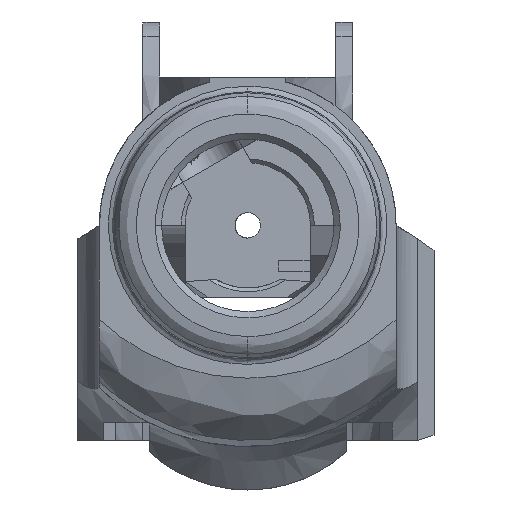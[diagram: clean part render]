
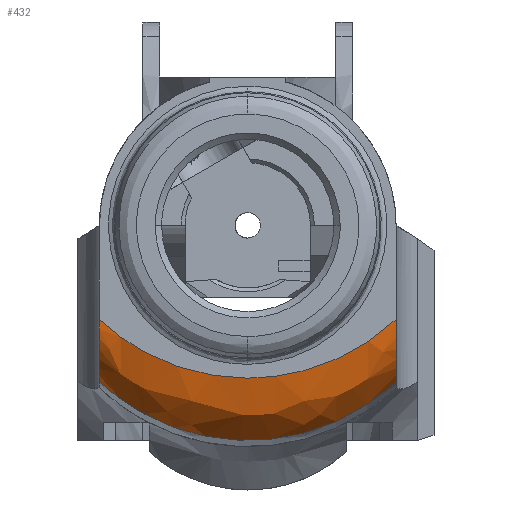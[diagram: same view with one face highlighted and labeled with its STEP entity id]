
A CAD part, left-side view. The second image highlights one B-rep face of the part: STEP entity #432.
In plain terms, the highlighted free-form (B-spline) face has degree [3, 3] with [4, 10] control points.
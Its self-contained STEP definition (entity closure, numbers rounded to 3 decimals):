
#432=ADVANCED_FACE('',(#892),#7309,.T.);
#892=FACE_OUTER_BOUND('',#1352,.T.);
#1352=EDGE_LOOP('',(#3797,#3798,#3799,#3800,#3801,#3802));
#3797=ORIENTED_EDGE('',*,*,#4130,.T.);
#3798=ORIENTED_EDGE('',*,*,#3877,.T.);
#3799=ORIENTED_EDGE('',*,*,#3878,.T.);
#3800=ORIENTED_EDGE('',*,*,#3879,.T.);
#3801=ORIENTED_EDGE('',*,*,#4136,.F.);
#3802=ORIENTED_EDGE('',*,*,#4133,.F.);
#3877=EDGE_CURVE('',#6382,#6383,#6224,.T.);
#3878=EDGE_CURVE('',#6383,#6384,#5129,.T.);
#3879=EDGE_CURVE('',#6384,#6385,#6225,.T.);
#4130=EDGE_CURVE('',#6630,#6382,#5347,.T.);
#4133=EDGE_CURVE('',#6630,#6631,#6259,.T.);
#4136=EDGE_CURVE('',#6631,#6385,#5352,.T.);
#5129=B_SPLINE_CURVE_WITH_KNOTS('',3,(#11458,#11459,#11460,#11461,#11462),
 .UNSPECIFIED.,.F.,.F.,(4,1,4),(0.,0.015,0.029),
 .UNSPECIFIED.);
#5347=B_SPLINE_CURVE_WITH_KNOTS('',3,(#12147,#12148,#12149,#12150,#12151,
#12152,#12153,#12154,#12155,#12156,#12157),.UNSPECIFIED.,.F.,.F.,(4,1,1,
1,1,1,1,1,4),(0.,0.77,1.54,2.311,3.081,
3.851,4.621,5.392,6.162),
 .UNSPECIFIED.);
#5352=B_SPLINE_CURVE_WITH_KNOTS('',3,(#12169,#12170,#12171,#12172,#12173,
#12174,#12175,#12176,#12177,#12178,#12179),.UNSPECIFIED.,.F.,.F.,(4,1,1,
1,1,1,1,1,4),(-6.162,-5.392,-4.621,-3.851,
-3.081,-2.311,-1.54,-0.77,
0.),.UNSPECIFIED.);
#6224=(
BOUNDED_CURVE()
B_SPLINE_CURVE(2,(#11455,#11456,#11457),.UNSPECIFIED.,.F.,.F.)
B_SPLINE_CURVE_WITH_KNOTS((3,3),(0.,12.819),.UNSPECIFIED.)
CURVE()
GEOMETRIC_REPRESENTATION_ITEM()
RATIONAL_B_SPLINE_CURVE((1.,0.93,1.))
REPRESENTATION_ITEM('')
);
#6225=(
BOUNDED_CURVE()
B_SPLINE_CURVE(2,(#11463,#11464,#11465),.UNSPECIFIED.,.F.,.F.)
B_SPLINE_CURVE_WITH_KNOTS((3,3),(0.,12.797),.UNSPECIFIED.)
CURVE()
GEOMETRIC_REPRESENTATION_ITEM()
RATIONAL_B_SPLINE_CURVE((1.,0.93,1.))
REPRESENTATION_ITEM('')
);
#6259=(
BOUNDED_CURVE()
B_SPLINE_CURVE(2,(#12162,#12163,#12164),.UNSPECIFIED.,.F.,.F.)
B_SPLINE_CURVE_WITH_KNOTS((3,3),(-25.645,0.),.UNSPECIFIED.)
CURVE()
GEOMETRIC_REPRESENTATION_ITEM()
RATIONAL_B_SPLINE_CURVE((1.,0.729,1.))
REPRESENTATION_ITEM('')
);
#6382=VERTEX_POINT('',#10638);
#6383=VERTEX_POINT('',#10639);
#6384=VERTEX_POINT('',#10640);
#6385=VERTEX_POINT('',#10641);
#6630=VERTEX_POINT('',#10886);
#6631=VERTEX_POINT('',#10887);
#7309=(
BOUNDED_SURFACE()
B_SPLINE_SURFACE(3,3,((#10475,#10476,#10477,#10478,#10479,#10480,#10481,
#10482,#10483,#10484),(#10485,#10486,#10487,#10488,#10489,#10490,#10491,
#10492,#10493,#10494),(#10495,#10496,#10497,#10498,#10499,#10500,#10501,
#10502,#10503,#10504),(#10505,#10506,#10507,#10508,#10509,#10510,#10511,
#10512,#10513,#10514)),.UNSPECIFIED.,.F.,.F.,.F.)
B_SPLINE_SURFACE_WITH_KNOTS((4,4),(4,1,1,1,1,1,1,4),(0.,29.83),
(0.,0.274,1.51,2.746,3.982,
5.218,6.455,6.728),.UNSPECIFIED.)
GEOMETRIC_REPRESENTATION_ITEM()
RATIONAL_B_SPLINE_SURFACE(((1.171,1.171,1.171,
1.171,1.171,1.171,1.171,1.171,
1.171,1.171),(0.943,0.943,0.943,
0.943,0.943,0.943,0.943,0.943,
0.943,0.943),(0.943,0.943,0.943,
0.943,0.943,0.943,0.943,0.943,
0.943,0.943),(1.171,1.171,1.171,
1.171,1.171,1.171,1.171,1.171,
1.171,1.171)))
REPRESENTATION_ITEM('')
SURFACE()
);
#10475=CARTESIAN_POINT('',(-128.892,12.009,68.471));
#10476=CARTESIAN_POINT('',(-128.976,12.009,68.505));
#10477=CARTESIAN_POINT('',(-129.437,12.009,68.701));
#10478=CARTESIAN_POINT('',(-130.222,12.009,69.173));
#10479=CARTESIAN_POINT('',(-131.113,12.009,70.032));
#10480=CARTESIAN_POINT('',(-131.787,12.009,71.07));
#10481=CARTESIAN_POINT('',(-132.211,12.009,72.232));
#10482=CARTESIAN_POINT('',(-132.323,12.009,73.142));
#10483=CARTESIAN_POINT('',(-132.316,12.009,73.643));
#10484=CARTESIAN_POINT('',(-132.312,12.009,73.733));
#10485=CARTESIAN_POINT('',(-128.892,4.972,61.447));
#10486=CARTESIAN_POINT('',(-128.976,4.972,61.48));
#10487=CARTESIAN_POINT('',(-129.437,4.972,61.677));
#10488=CARTESIAN_POINT('',(-130.222,4.972,62.148));
#10489=CARTESIAN_POINT('',(-131.113,4.972,63.008));
#10490=CARTESIAN_POINT('',(-131.787,4.972,64.046));
#10491=CARTESIAN_POINT('',(-132.211,4.972,65.208));
#10492=CARTESIAN_POINT('',(-132.323,4.972,66.118));
#10493=CARTESIAN_POINT('',(-132.316,4.972,66.618));
#10494=CARTESIAN_POINT('',(-132.312,4.972,66.709));
#10495=CARTESIAN_POINT('',(-128.892,-4.972,61.447));
#10496=CARTESIAN_POINT('',(-128.976,-4.972,61.48));
#10497=CARTESIAN_POINT('',(-129.437,-4.972,61.677));
#10498=CARTESIAN_POINT('',(-130.222,-4.972,62.148));
#10499=CARTESIAN_POINT('',(-131.113,-4.972,63.008));
#10500=CARTESIAN_POINT('',(-131.787,-4.972,64.046));
#10501=CARTESIAN_POINT('',(-132.211,-4.972,65.208));
#10502=CARTESIAN_POINT('',(-132.323,-4.972,66.118));
#10503=CARTESIAN_POINT('',(-132.316,-4.972,66.618));
#10504=CARTESIAN_POINT('',(-132.312,-4.972,66.709));
#10505=CARTESIAN_POINT('',(-128.892,-12.009,68.471));
#10506=CARTESIAN_POINT('',(-128.976,-12.009,68.505));
#10507=CARTESIAN_POINT('',(-129.437,-12.009,68.701));
#10508=CARTESIAN_POINT('',(-130.222,-12.009,69.173));
#10509=CARTESIAN_POINT('',(-131.113,-12.009,70.032));
#10510=CARTESIAN_POINT('',(-131.787,-12.009,71.07));
#10511=CARTESIAN_POINT('',(-132.211,-12.009,72.232));
#10512=CARTESIAN_POINT('',(-132.323,-12.009,73.142));
#10513=CARTESIAN_POINT('',(-132.316,-12.009,73.643));
#10514=CARTESIAN_POINT('',(-132.312,-12.009,73.733));
#10638=CARTESIAN_POINT('',(-132.316,-11.641,73.104));
#10639=CARTESIAN_POINT('',(-132.316,-0.004,68.493));
#10640=CARTESIAN_POINT('',(-132.316,0.026,68.493));
#10641=CARTESIAN_POINT('',(-132.316,11.641,73.104));
#10886=CARTESIAN_POINT('',(-129.142,-11.641,68.221));
#10887=CARTESIAN_POINT('',(-129.142,11.641,68.221));
#11455=CARTESIAN_POINT('',(-132.316,-11.641,73.104));
#11456=CARTESIAN_POINT('',(-132.316,-6.735,68.495));
#11457=CARTESIAN_POINT('',(-132.316,-0.004,68.493));
#11458=CARTESIAN_POINT('',(-132.316,-0.004,68.493));
#11459=CARTESIAN_POINT('',(-132.316,0.002,68.493));
#11460=CARTESIAN_POINT('',(-132.316,0.012,68.493));
#11461=CARTESIAN_POINT('',(-132.316,0.021,68.493));
#11462=CARTESIAN_POINT('',(-132.316,0.026,68.493));
#11463=CARTESIAN_POINT('',(-132.316,0.026,68.493));
#11464=CARTESIAN_POINT('',(-132.316,6.744,68.503));
#11465=CARTESIAN_POINT('',(-132.316,11.641,73.104));
#12147=CARTESIAN_POINT('',(-129.142,-11.641,68.221));
#12148=CARTESIAN_POINT('',(-129.376,-11.641,68.328));
#12149=CARTESIAN_POINT('',(-129.824,-11.641,68.572));
#12150=CARTESIAN_POINT('',(-130.444,-11.641,69.033));
#12151=CARTESIAN_POINT('',(-130.991,-11.641,69.576));
#12152=CARTESIAN_POINT('',(-131.456,-11.641,70.192));
#12153=CARTESIAN_POINT('',(-131.829,-11.641,70.866));
#12154=CARTESIAN_POINT('',(-132.103,-11.641,71.587));
#12155=CARTESIAN_POINT('',(-132.272,-11.641,72.338));
#12156=CARTESIAN_POINT('',(-132.314,-11.641,72.847));
#12157=CARTESIAN_POINT('',(-132.316,-11.641,73.104));
#12162=CARTESIAN_POINT('',(-129.142,-11.641,68.221));
#12163=CARTESIAN_POINT('',(-129.142,0.,57.283));
#12164=CARTESIAN_POINT('',(-129.142,11.641,68.221));
#12169=CARTESIAN_POINT('',(-129.142,11.641,68.221));
#12170=CARTESIAN_POINT('',(-129.376,11.641,68.328));
#12171=CARTESIAN_POINT('',(-129.824,11.641,68.572));
#12172=CARTESIAN_POINT('',(-130.444,11.641,69.033));
#12173=CARTESIAN_POINT('',(-130.991,11.641,69.576));
#12174=CARTESIAN_POINT('',(-131.456,11.641,70.192));
#12175=CARTESIAN_POINT('',(-131.829,11.641,70.866));
#12176=CARTESIAN_POINT('',(-132.103,11.641,71.587));
#12177=CARTESIAN_POINT('',(-132.272,11.641,72.338));
#12178=CARTESIAN_POINT('',(-132.314,11.641,72.847));
#12179=CARTESIAN_POINT('',(-132.316,11.641,73.104));
